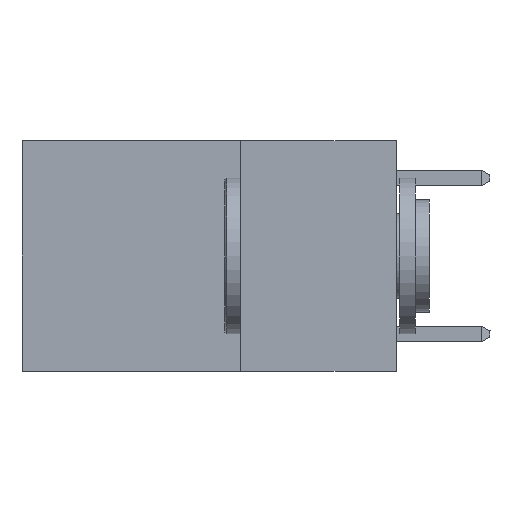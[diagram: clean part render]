
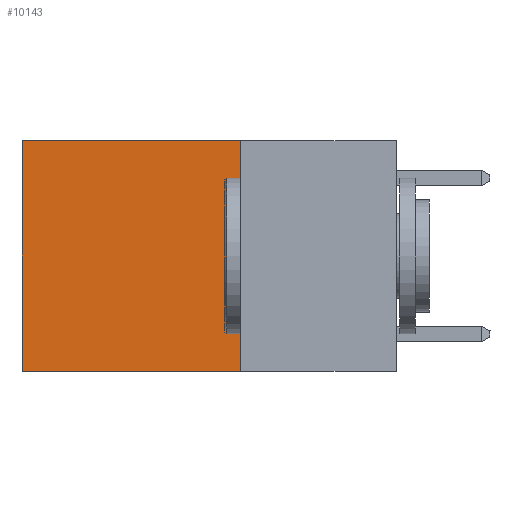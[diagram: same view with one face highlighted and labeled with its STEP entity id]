
A CAD part, left-side view. The second image highlights one B-rep face of the part: STEP entity #10143.
In plain terms, the highlighted planar face has unit normal (-1, 0, 0).
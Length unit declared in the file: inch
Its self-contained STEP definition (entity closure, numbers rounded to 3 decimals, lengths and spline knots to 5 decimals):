
#96 = EDGE_CURVE ( 'NONE', #10790, #4322, #6129, .T. ) ;
#867 = AXIS2_PLACEMENT_3D ( 'NONE', #1834, #4365, #10097 ) ;
#1099 = ORIENTED_EDGE ( 'NONE', *, *, #1297, .T. ) ;
#1139 = VECTOR ( 'NONE', #7579, 39.37008 ) ;
#1297 = EDGE_CURVE ( 'NONE', #4774, #2371, #8074, .T. ) ;
#1834 = CARTESIAN_POINT ( 'NONE',  ( 0.2625, 0.25, 0. ) ) ;
#2050 = DIRECTION ( 'NONE',  ( 0., 1., 0. ) ) ;
#2309 = CARTESIAN_POINT ( 'NONE',  ( 0.2625, 0.25, 0. ) ) ;
#2371 = VERTEX_POINT ( 'NONE', #4894 ) ;
#3223 = CARTESIAN_POINT ( 'NONE',  ( 0.2625, 0.25, 0. ) ) ;
#3541 = PLANE ( 'NONE',  #867 ) ;
#3645 = VECTOR ( 'NONE', #2050, 39.37008 ) ;
#3672 = CARTESIAN_POINT ( 'NONE',  ( 0.2625, 0.25, -0.37 ) ) ;
#3859 = VECTOR ( 'NONE', #3867, 39.37008 ) ;
#3867 = DIRECTION ( 'NONE',  ( 0., 1., 0. ) ) ;
#4322 = VERTEX_POINT ( 'NONE', #10490 ) ;
#4365 = DIRECTION ( 'NONE',  ( 1., 0., 0. ) ) ;
#4774 = VERTEX_POINT ( 'NONE', #7842 ) ;
#4850 = EDGE_CURVE ( 'NONE', #2371, #4322, #5716, .T. ) ;
#4894 = CARTESIAN_POINT ( 'NONE',  ( 0.2625, 0.6, 0. ) ) ;
#5300 = CARTESIAN_POINT ( 'NONE',  ( 0.2625, 0.25, -0.37 ) ) ;
#5627 = LINE ( 'NONE', #2309, #7808 ) ;
#5716 = LINE ( 'NONE', #7581, #1139 ) ;
#5813 = ORIENTED_EDGE ( 'NONE', *, *, #9385, .F. ) ;
#5864 = FACE_OUTER_BOUND ( 'NONE', #8770, .T. ) ;
#6129 = LINE ( 'NONE', #3672, #3859 ) ;
#7579 = DIRECTION ( 'NONE',  ( 0., 0., -1. ) ) ;
#7581 = CARTESIAN_POINT ( 'NONE',  ( 0.2625, 0.6, 0. ) ) ;
#7808 = VECTOR ( 'NONE', #8134, 39.37008 ) ;
#7842 = CARTESIAN_POINT ( 'NONE',  ( 0.2625, 0.25, 0. ) ) ;
#7947 = ORIENTED_EDGE ( 'NONE', *, *, #96, .F. ) ;
#8074 = LINE ( 'NONE', #3223, #3645 ) ;
#8134 = DIRECTION ( 'NONE',  ( 0., 0., -1. ) ) ;
#8770 = EDGE_LOOP ( 'NONE', ( #9521, #7947, #5813, #1099 ) ) ;
#9385 = EDGE_CURVE ( 'NONE', #4774, #10790, #5627, .T. ) ;
#9521 = ORIENTED_EDGE ( 'NONE', *, *, #4850, .T. ) ;
#10097 = DIRECTION ( 'NONE',  ( 0., 0., -1. ) ) ;
#10143 = ADVANCED_FACE ( 'NONE', ( #5864 ), #3541, .F. ) ;
#10490 = CARTESIAN_POINT ( 'NONE',  ( 0.2625, 0.6, -0.37 ) ) ;
#10790 = VERTEX_POINT ( 'NONE', #5300 ) ;
